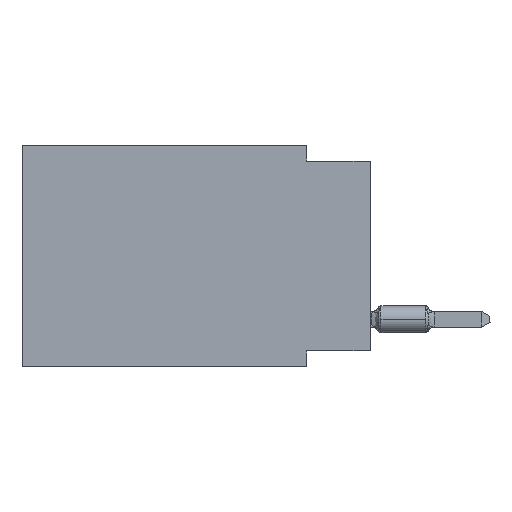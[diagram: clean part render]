
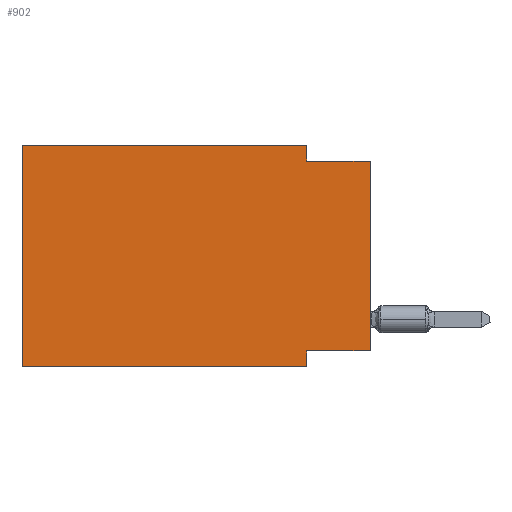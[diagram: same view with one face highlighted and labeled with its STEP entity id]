
A CAD part, left-side view. The second image highlights one B-rep face of the part: STEP entity #902.
In plain terms, the highlighted planar face has unit normal (-1, 0, 0).
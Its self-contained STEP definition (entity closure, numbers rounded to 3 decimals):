
#902 = ADVANCED_FACE ( 'NONE', ( #37303 ), #8694, .F. ) ;
#2844 = DIRECTION ( 'NONE',  ( 1., 0., 0. ) ) ;
#2915 = VECTOR ( 'NONE', #38145, 1000. ) ;
#2991 = LINE ( 'NONE', #31600, #40722 ) ;
#3099 = LINE ( 'NONE', #28982, #31779 ) ;
#4807 = ORIENTED_EDGE ( 'NONE', *, *, #12672, .F. ) ;
#5787 = DIRECTION ( 'NONE',  ( 0., 0., -1. ) ) ;
#6495 = ORIENTED_EDGE ( 'NONE', *, *, #38757, .T. ) ;
#6775 = CARTESIAN_POINT ( 'NONE',  ( 0., 2.54, -0.635 ) ) ;
#6797 = CARTESIAN_POINT ( 'NONE',  ( 0., 13.97, -8.89 ) ) ;
#7171 = VERTEX_POINT ( 'NONE', #17577 ) ;
#7657 = DIRECTION ( 'NONE',  ( 0., -1., 0. ) ) ;
#8663 = VERTEX_POINT ( 'NONE', #34829 ) ;
#8694 = PLANE ( 'NONE',  #33686 ) ;
#9570 = VECTOR ( 'NONE', #7657, 1000. ) ;
#9893 = DIRECTION ( 'NONE',  ( 0., -1., 0. ) ) ;
#9943 = VECTOR ( 'NONE', #16817, 1000. ) ;
#10344 = CARTESIAN_POINT ( 'NONE',  ( 0., 2.54, 0. ) ) ;
#12138 = ORIENTED_EDGE ( 'NONE', *, *, #25887, .F. ) ;
#12672 = EDGE_CURVE ( 'NONE', #16273, #27668, #35827, .T. ) ;
#13046 = LINE ( 'NONE', #6797, #16709 ) ;
#14188 = CARTESIAN_POINT ( 'NONE',  ( 0., 0., -8.255 ) ) ;
#14318 = CARTESIAN_POINT ( 'NONE',  ( 0., 13.97, 0. ) ) ;
#14766 = DIRECTION ( 'NONE',  ( 0., 0., -1. ) ) ;
#14818 = VERTEX_POINT ( 'NONE', #27013 ) ;
#16273 = VERTEX_POINT ( 'NONE', #25905 ) ;
#16448 = DIRECTION ( 'NONE',  ( 0., -1., 0. ) ) ;
#16709 = VECTOR ( 'NONE', #9893, 1000. ) ;
#16747 = EDGE_CURVE ( 'NONE', #26676, #16273, #39982, .T. ) ;
#16751 = VERTEX_POINT ( 'NONE', #17232 ) ;
#16817 = DIRECTION ( 'NONE',  ( 0., 0., -1. ) ) ;
#17232 = CARTESIAN_POINT ( 'NONE',  ( 0., 2.54, -8.89 ) ) ;
#17577 = CARTESIAN_POINT ( 'NONE',  ( 0., 0., -8.255 ) ) ;
#19053 = EDGE_CURVE ( 'NONE', #7171, #14818, #25197, .T. ) ;
#21642 = CARTESIAN_POINT ( 'NONE',  ( 0., 13.97, 0. ) ) ;
#22093 = EDGE_CURVE ( 'NONE', #8663, #16751, #27512, .T. ) ;
#22448 = CARTESIAN_POINT ( 'NONE',  ( 0., 13.97, 0. ) ) ;
#25197 = LINE ( 'NONE', #37537, #2915 ) ;
#25887 = EDGE_CURVE ( 'NONE', #30443, #26676, #2991, .T. ) ;
#25905 = CARTESIAN_POINT ( 'NONE',  ( 0., 2.54, 0. ) ) ;
#26676 = VERTEX_POINT ( 'NONE', #22448 ) ;
#27013 = CARTESIAN_POINT ( 'NONE',  ( 0., 0., -0.635 ) ) ;
#27512 = LINE ( 'NONE', #30631, #32707 ) ;
#27668 = VERTEX_POINT ( 'NONE', #6775 ) ;
#27831 = ORIENTED_EDGE ( 'NONE', *, *, #22093, .F. ) ;
#28181 = ORIENTED_EDGE ( 'NONE', *, *, #39980, .F. ) ;
#28982 = CARTESIAN_POINT ( 'NONE',  ( 0., 0., -0.635 ) ) ;
#29846 = DIRECTION ( 'NONE',  ( 0., 1., 0. ) ) ;
#30442 = VECTOR ( 'NONE', #29846, 1000. ) ;
#30443 = VERTEX_POINT ( 'NONE', #40423 ) ;
#30631 = CARTESIAN_POINT ( 'NONE',  ( 0., 2.54, -8.89 ) ) ;
#31600 = CARTESIAN_POINT ( 'NONE',  ( 0., 13.97, 0. ) ) ;
#31779 = VECTOR ( 'NONE', #16448, 1000. ) ;
#32418 = DIRECTION ( 'NONE',  ( 0., 0., 1. ) ) ;
#32550 = ORIENTED_EDGE ( 'NONE', *, *, #39770, .F. ) ;
#32707 = VECTOR ( 'NONE', #14766, 1000. ) ;
#33390 = LINE ( 'NONE', #14188, #30442 ) ;
#33686 = AXIS2_PLACEMENT_3D ( 'NONE', #21642, #2844, #5787 ) ;
#34292 = EDGE_LOOP ( 'NONE', ( #34739, #28181, #4807, #36463, #12138, #6495, #27831, #32550 ) ) ;
#34739 = ORIENTED_EDGE ( 'NONE', *, *, #19053, .T. ) ;
#34829 = CARTESIAN_POINT ( 'NONE',  ( 0., 2.54, -8.255 ) ) ;
#35827 = LINE ( 'NONE', #10344, #9943 ) ;
#36463 = ORIENTED_EDGE ( 'NONE', *, *, #16747, .F. ) ;
#37303 = FACE_OUTER_BOUND ( 'NONE', #34292, .T. ) ;
#37537 = CARTESIAN_POINT ( 'NONE',  ( 0., 0., 0. ) ) ;
#38145 = DIRECTION ( 'NONE',  ( 0., 0., 1. ) ) ;
#38757 = EDGE_CURVE ( 'NONE', #30443, #16751, #13046, .T. ) ;
#39770 = EDGE_CURVE ( 'NONE', #7171, #8663, #33390, .T. ) ;
#39980 = EDGE_CURVE ( 'NONE', #27668, #14818, #3099, .T. ) ;
#39982 = LINE ( 'NONE', #14318, #9570 ) ;
#40423 = CARTESIAN_POINT ( 'NONE',  ( 0., 13.97, -8.89 ) ) ;
#40722 = VECTOR ( 'NONE', #32418, 1000. ) ;
